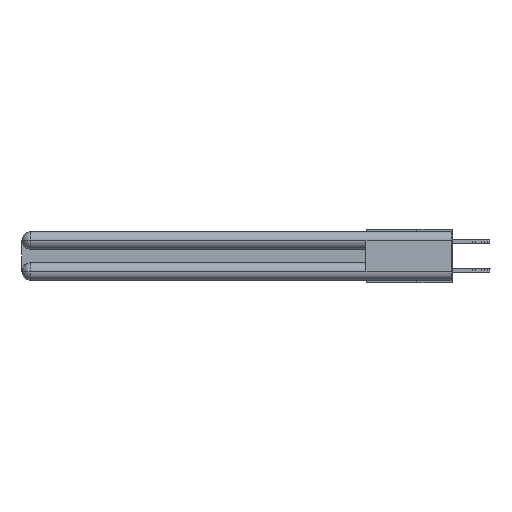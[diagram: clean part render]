
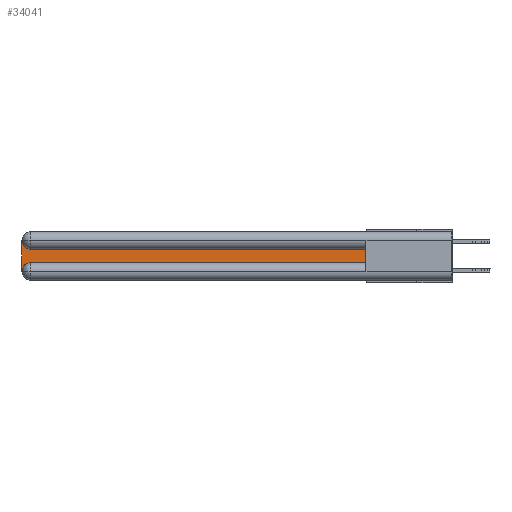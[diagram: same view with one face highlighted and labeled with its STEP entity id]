
A CAD part, left-side view. The second image highlights one B-rep face of the part: STEP entity #34041.
In plain terms, the highlighted planar face has unit normal (-1, 0, 0).
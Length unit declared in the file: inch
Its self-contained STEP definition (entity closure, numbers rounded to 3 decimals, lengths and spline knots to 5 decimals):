
#774 = CARTESIAN_POINT ( 'NONE',  ( 0.075, 3., -0.2775 ) ) ;
#1603 = DIRECTION ( 'NONE',  ( 0., 0., -1. ) ) ;
#5004 = CIRCLE ( 'NONE', #21241, 0.06 ) ;
#5420 = LINE ( 'NONE', #19059, #23981 ) ;
#5670 = AXIS2_PLACEMENT_3D ( 'NONE', #23956, #21428, #10709 ) ;
#6075 = ORIENTED_EDGE ( 'NONE', *, *, #15999, .T. ) ;
#6629 = PLANE ( 'NONE',  #14194 ) ;
#6749 = DIRECTION ( 'NONE',  ( 0., 0., -1. ) ) ;
#7652 = ORIENTED_EDGE ( 'NONE', *, *, #12596, .T. ) ;
#7805 = DIRECTION ( 'NONE',  ( 0., -1., 0. ) ) ;
#8976 = EDGE_CURVE ( 'NONE', #25210, #24789, #5420, .T. ) ;
#10176 = VECTOR ( 'NONE', #24390, 39.37008 ) ;
#10381 = EDGE_LOOP ( 'NONE', ( #29412, #7652, #13390, #6075, #28538, #35458 ) ) ;
#10709 = DIRECTION ( 'NONE',  ( 0., 0., -1. ) ) ;
#12222 = CARTESIAN_POINT ( 'NONE',  ( 0.075, 3., -0.1225 ) ) ;
#12458 = DIRECTION ( 'NONE',  ( 1., 0., 0. ) ) ;
#12596 = EDGE_CURVE ( 'NONE', #18181, #18487, #21051, .T. ) ;
#13390 = ORIENTED_EDGE ( 'NONE', *, *, #14295, .T. ) ;
#13637 = CARTESIAN_POINT ( 'NONE',  ( 0.075, 0.6, -0.1225 ) ) ;
#14065 = EDGE_CURVE ( 'NONE', #24789, #18181, #30028, .T. ) ;
#14194 = AXIS2_PLACEMENT_3D ( 'NONE', #12222, #12458, #6749 ) ;
#14295 = EDGE_CURVE ( 'NONE', #18487, #16964, #29151, .T. ) ;
#14706 = EDGE_CURVE ( 'NONE', #32849, #25210, #23887, .T. ) ;
#14859 = DIRECTION ( 'NONE',  ( 0., 0., -1. ) ) ;
#15999 = EDGE_CURVE ( 'NONE', #16964, #32849, #5004, .T. ) ;
#16015 = CARTESIAN_POINT ( 'NONE',  ( 0.075, 0.6, -0.2175 ) ) ;
#16964 = VERTEX_POINT ( 'NONE', #774 ) ;
#18181 = VERTEX_POINT ( 'NONE', #28687 ) ;
#18487 = VERTEX_POINT ( 'NONE', #25287 ) ;
#19059 = CARTESIAN_POINT ( 'NONE',  ( 0.075, 0.6, -0.2175 ) ) ;
#20179 = CARTESIAN_POINT ( 'NONE',  ( 0.075, 3., -0.2175 ) ) ;
#20699 = FACE_OUTER_BOUND ( 'NONE', #10381, .T. ) ;
#20847 = CARTESIAN_POINT ( 'NONE',  ( 0.075, 2.94, -0.2175 ) ) ;
#21051 = CIRCLE ( 'NONE', #5670, 0.06 ) ;
#21241 = AXIS2_PLACEMENT_3D ( 'NONE', #31802, #23676, #1603 ) ;
#21299 = VECTOR ( 'NONE', #7805, 39.37008 ) ;
#21428 = DIRECTION ( 'NONE',  ( 1., 0., 0. ) ) ;
#21763 = VECTOR ( 'NONE', #14859, 39.37008 ) ;
#23676 = DIRECTION ( 'NONE',  ( 1., 0., 0. ) ) ;
#23887 = LINE ( 'NONE', #16015, #21299 ) ;
#23956 = CARTESIAN_POINT ( 'NONE',  ( 0.075, 2.94, -0.0625 ) ) ;
#23981 = VECTOR ( 'NONE', #30174, 39.37008 ) ;
#24390 = DIRECTION ( 'NONE',  ( 0., 1., 0. ) ) ;
#24789 = VERTEX_POINT ( 'NONE', #13637 ) ;
#25210 = VERTEX_POINT ( 'NONE', #34884 ) ;
#25287 = CARTESIAN_POINT ( 'NONE',  ( 0.075, 3., -0.0625 ) ) ;
#27429 = CARTESIAN_POINT ( 'NONE',  ( 0.075, 0.6, -0.1225 ) ) ;
#28538 = ORIENTED_EDGE ( 'NONE', *, *, #14706, .T. ) ;
#28687 = CARTESIAN_POINT ( 'NONE',  ( 0.075, 2.94, -0.1225 ) ) ;
#29151 = LINE ( 'NONE', #20179, #21763 ) ;
#29412 = ORIENTED_EDGE ( 'NONE', *, *, #14065, .T. ) ;
#30028 = LINE ( 'NONE', #27429, #10176 ) ;
#30174 = DIRECTION ( 'NONE',  ( 0., 0., 1. ) ) ;
#31802 = CARTESIAN_POINT ( 'NONE',  ( 0.075, 2.94, -0.2775 ) ) ;
#32849 = VERTEX_POINT ( 'NONE', #20847 ) ;
#34041 = ADVANCED_FACE ( 'NONE', ( #20699 ), #6629, .F. ) ;
#34884 = CARTESIAN_POINT ( 'NONE',  ( 0.075, 0.6, -0.2175 ) ) ;
#35458 = ORIENTED_EDGE ( 'NONE', *, *, #8976, .T. ) ;
